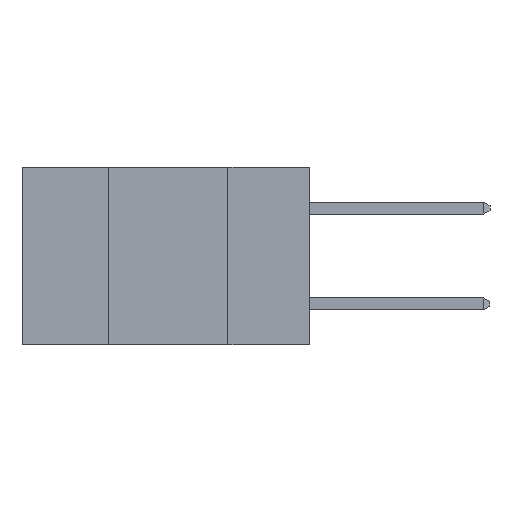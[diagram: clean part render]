
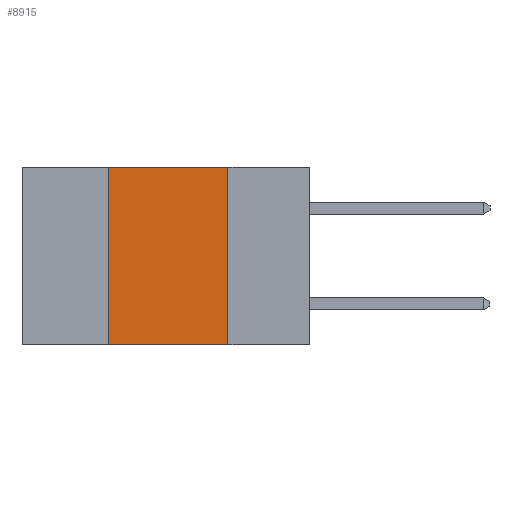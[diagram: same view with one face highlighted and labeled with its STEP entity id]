
A CAD part, left-side view. The second image highlights one B-rep face of the part: STEP entity #8915.
In plain terms, the highlighted planar face has unit normal (-1, 0, 0).
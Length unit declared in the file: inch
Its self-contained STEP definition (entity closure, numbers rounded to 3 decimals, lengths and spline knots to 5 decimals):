
#174 = VERTEX_POINT ( 'NONE', #7760 ) ;
#410 = DIRECTION ( 'NONE',  ( 0., -1., 0. ) ) ;
#1057 = PLANE ( 'NONE',  #1716 ) ;
#1079 = VECTOR ( 'NONE', #410, 39.37008 ) ;
#1270 = CARTESIAN_POINT ( 'NONE',  ( 0., 0.42, 0. ) ) ;
#1716 = AXIS2_PLACEMENT_3D ( 'NONE', #3958, #3090, #6855 ) ;
#2145 = VECTOR ( 'NONE', #6921, 39.37008 ) ;
#2525 = LINE ( 'NONE', #3892, #1079 ) ;
#2982 = EDGE_CURVE ( 'NONE', #6036, #3736, #5833, .T. ) ;
#3014 = ORIENTED_EDGE ( 'NONE', *, *, #8152, .F. ) ;
#3090 = DIRECTION ( 'NONE',  ( 1., 0., 0. ) ) ;
#3542 = LINE ( 'NONE', #1270, #3715 ) ;
#3715 = VECTOR ( 'NONE', #4224, 39.37008 ) ;
#3736 = VERTEX_POINT ( 'NONE', #7013 ) ;
#3803 = ORIENTED_EDGE ( 'NONE', *, *, #7340, .F. ) ;
#3892 = CARTESIAN_POINT ( 'NONE',  ( 0., 0.6, 0. ) ) ;
#3958 = CARTESIAN_POINT ( 'NONE',  ( 0., 0.6, 0. ) ) ;
#4070 = LINE ( 'NONE', #7787, #2145 ) ;
#4224 = DIRECTION ( 'NONE',  ( 0., 0., 1. ) ) ;
#5111 = ORIENTED_EDGE ( 'NONE', *, *, #8207, .F. ) ;
#5367 = EDGE_LOOP ( 'NONE', ( #3803, #3014, #5111, #9373 ) ) ;
#5833 = LINE ( 'NONE', #7279, #6207 ) ;
#6036 = VERTEX_POINT ( 'NONE', #9490 ) ;
#6207 = VECTOR ( 'NONE', #8192, 39.37008 ) ;
#6709 = FACE_OUTER_BOUND ( 'NONE', #5367, .T. ) ;
#6855 = DIRECTION ( 'NONE',  ( 0., 0., -1. ) ) ;
#6921 = DIRECTION ( 'NONE',  ( 0., 0., -1. ) ) ;
#7013 = CARTESIAN_POINT ( 'NONE',  ( 0., 0.17, -0.37 ) ) ;
#7279 = CARTESIAN_POINT ( 'NONE',  ( 0., 0.6, -0.37 ) ) ;
#7340 = EDGE_CURVE ( 'NONE', #174, #3736, #4070, .T. ) ;
#7760 = CARTESIAN_POINT ( 'NONE',  ( 0., 0.17, 0. ) ) ;
#7787 = CARTESIAN_POINT ( 'NONE',  ( 0., 0.17, 0. ) ) ;
#8036 = CARTESIAN_POINT ( 'NONE',  ( 0., 0.42, 0. ) ) ;
#8152 = EDGE_CURVE ( 'NONE', #8348, #174, #2525, .T. ) ;
#8192 = DIRECTION ( 'NONE',  ( 0., -1., 0. ) ) ;
#8207 = EDGE_CURVE ( 'NONE', #6036, #8348, #3542, .T. ) ;
#8348 = VERTEX_POINT ( 'NONE', #8036 ) ;
#8915 = ADVANCED_FACE ( 'NONE', ( #6709 ), #1057, .F. ) ;
#9373 = ORIENTED_EDGE ( 'NONE', *, *, #2982, .T. ) ;
#9490 = CARTESIAN_POINT ( 'NONE',  ( 0., 0.42, -0.37 ) ) ;
